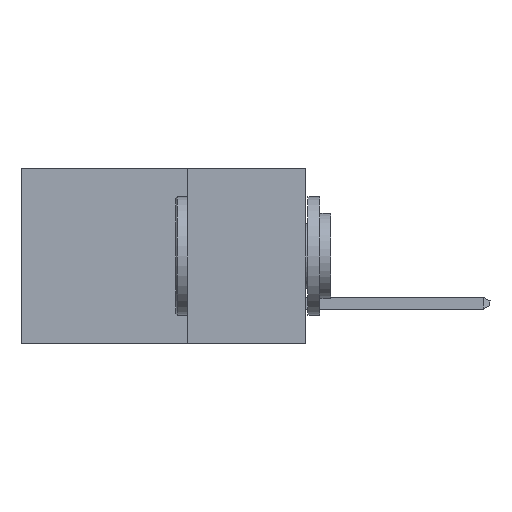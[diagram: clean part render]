
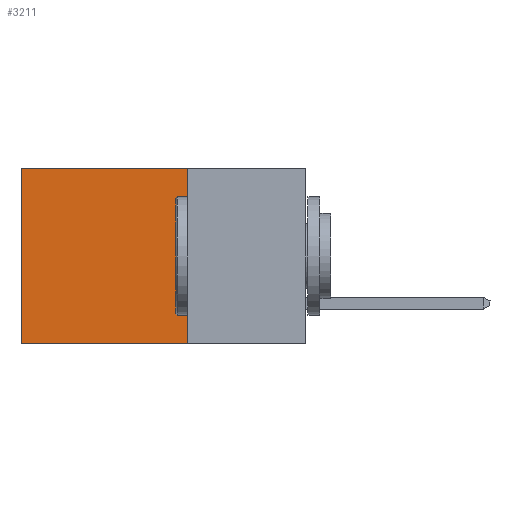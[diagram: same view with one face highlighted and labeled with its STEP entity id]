
A CAD part, left-side view. The second image highlights one B-rep face of the part: STEP entity #3211.
In plain terms, the highlighted planar face has unit normal (-1, 0, 0).
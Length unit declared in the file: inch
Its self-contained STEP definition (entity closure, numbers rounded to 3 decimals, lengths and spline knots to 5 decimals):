
#18 = CARTESIAN_POINT ( 'NONE',  ( 0.2615, 0.6, 0. ) ) ;
#735 = CARTESIAN_POINT ( 'NONE',  ( 0.2615, 0.25, -0.37 ) ) ;
#736 = EDGE_CURVE ( 'NONE', #5614, #6436, #8935, .T. ) ;
#1046 = DIRECTION ( 'NONE',  ( 0., 1., 0. ) ) ;
#1083 = ORIENTED_EDGE ( 'NONE', *, *, #5447, .F. ) ;
#1573 = CARTESIAN_POINT ( 'NONE',  ( 0.2615, 0.6, -0.37 ) ) ;
#1656 = VECTOR ( 'NONE', #6222, 39.37008 ) ;
#1699 = ORIENTED_EDGE ( 'NONE', *, *, #2062, .T. ) ;
#2062 = EDGE_CURVE ( 'NONE', #4910, #5614, #7445, .T. ) ;
#2089 = VECTOR ( 'NONE', #4855, 39.37008 ) ;
#2441 = CARTESIAN_POINT ( 'NONE',  ( 0.2615, 0.25, 0. ) ) ;
#2816 = ORIENTED_EDGE ( 'NONE', *, *, #3546, .F. ) ;
#2852 = CARTESIAN_POINT ( 'NONE',  ( 0.2615, 0.25, 0. ) ) ;
#3031 = DIRECTION ( 'NONE',  ( 0., 1., 0. ) ) ;
#3211 = ADVANCED_FACE ( 'NONE', ( #8846 ), #6979, .F. ) ;
#3415 = VERTEX_POINT ( 'NONE', #4732 ) ;
#3546 = EDGE_CURVE ( 'NONE', #4910, #3415, #9387, .T. ) ;
#4732 = CARTESIAN_POINT ( 'NONE',  ( 0.2615, 0.25, -0.37 ) ) ;
#4855 = DIRECTION ( 'NONE',  ( 0., 0., -1. ) ) ;
#4910 = VERTEX_POINT ( 'NONE', #2441 ) ;
#5313 = LINE ( 'NONE', #735, #10451 ) ;
#5357 = AXIS2_PLACEMENT_3D ( 'NONE', #8069, #11734, #11556 ) ;
#5447 = EDGE_CURVE ( 'NONE', #3415, #6436, #5313, .T. ) ;
#5614 = VERTEX_POINT ( 'NONE', #18 ) ;
#6222 = DIRECTION ( 'NONE',  ( 0., 0., -1. ) ) ;
#6436 = VERTEX_POINT ( 'NONE', #11100 ) ;
#6871 = VECTOR ( 'NONE', #3031, 39.37008 ) ;
#6979 = PLANE ( 'NONE',  #5357 ) ;
#7445 = LINE ( 'NONE', #2852, #6871 ) ;
#7765 = CARTESIAN_POINT ( 'NONE',  ( 0.2615, 0.25, -0.37 ) ) ;
#8069 = CARTESIAN_POINT ( 'NONE',  ( 0.2615, 0.25, -0.37 ) ) ;
#8463 = ORIENTED_EDGE ( 'NONE', *, *, #736, .T. ) ;
#8846 = FACE_OUTER_BOUND ( 'NONE', #9247, .T. ) ;
#8935 = LINE ( 'NONE', #1573, #1656 ) ;
#9247 = EDGE_LOOP ( 'NONE', ( #8463, #1083, #2816, #1699 ) ) ;
#9387 = LINE ( 'NONE', #7765, #2089 ) ;
#10451 = VECTOR ( 'NONE', #1046, 39.37008 ) ;
#11100 = CARTESIAN_POINT ( 'NONE',  ( 0.2615, 0.6, -0.37 ) ) ;
#11556 = DIRECTION ( 'NONE',  ( 0., 0., -1. ) ) ;
#11734 = DIRECTION ( 'NONE',  ( 1., 0., 0. ) ) ;
